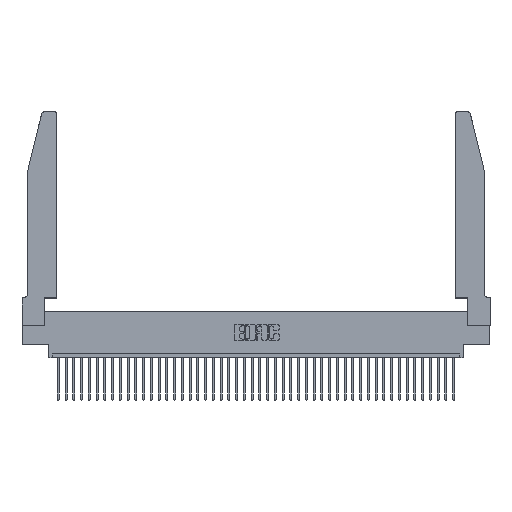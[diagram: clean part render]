
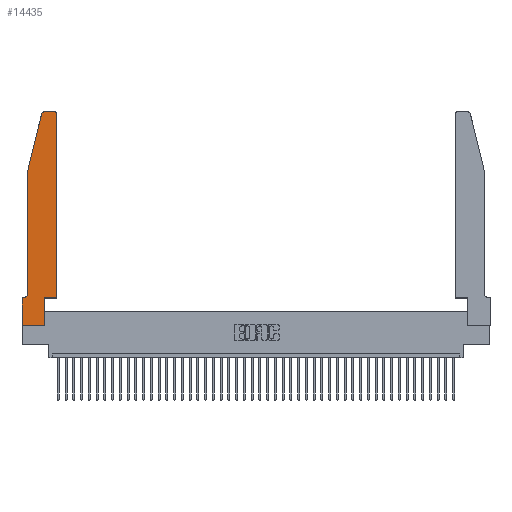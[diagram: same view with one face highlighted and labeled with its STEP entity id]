
A CAD part, top view. The second image highlights one B-rep face of the part: STEP entity #14435.
In plain terms, the highlighted planar face has unit normal (0, 0, 1).
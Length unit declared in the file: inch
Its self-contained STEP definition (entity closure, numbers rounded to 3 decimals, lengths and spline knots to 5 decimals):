
#172 = EDGE_CURVE ( 'NONE', #4846, #11020, #39690, .T. ) ;
#208 = VERTEX_POINT ( 'NONE', #11036 ) ;
#257 = VECTOR ( 'NONE', #23914, 39.37008 ) ;
#631 = VERTEX_POINT ( 'NONE', #15669 ) ;
#671 = EDGE_CURVE ( 'NONE', #29893, #631, #23609, .T. ) ;
#2301 = DIRECTION ( 'NONE',  ( -0.239, -0.971, 0. ) ) ;
#2379 = ORIENTED_EDGE ( 'NONE', *, *, #10121, .T. ) ;
#4210 = ORIENTED_EDGE ( 'NONE', *, *, #8724, .T. ) ;
#4527 = VERTEX_POINT ( 'NONE', #11928 ) ;
#4846 = VERTEX_POINT ( 'NONE', #10157 ) ;
#6494 = ORIENTED_EDGE ( 'NONE', *, *, #36489, .T. ) ;
#6908 = LINE ( 'NONE', #10457, #257 ) ;
#7983 = DIRECTION ( 'NONE',  ( -1., 0., 0. ) ) ;
#8712 = CARTESIAN_POINT ( 'NONE',  ( 0.0755, 2., 0.37 ) ) ;
#8724 = EDGE_CURVE ( 'NONE', #26366, #36573, #6908, .T. ) ;
#9397 = LINE ( 'NONE', #18089, #25946 ) ;
#9433 = EDGE_CURVE ( 'NONE', #10110, #4846, #27962, .T. ) ;
#10110 = VERTEX_POINT ( 'NONE', #39055 ) ;
#10121 = EDGE_CURVE ( 'NONE', #208, #10110, #38764, .T. ) ;
#10157 = CARTESIAN_POINT ( 'NONE',  ( 0., 0.35, 0.37 ) ) ;
#10457 = CARTESIAN_POINT ( 'NONE',  ( 0.4505, 0.35, 0.37 ) ) ;
#11008 = DIRECTION ( 'NONE',  ( 0., -1., 0. ) ) ;
#11020 = VERTEX_POINT ( 'NONE', #35320 ) ;
#11036 = CARTESIAN_POINT ( 'NONE',  ( 0.0755, 0.42, 0.37 ) ) ;
#11437 = CARTESIAN_POINT ( 'NONE',  ( 0.284, 2.72, 0.37 ) ) ;
#11928 = CARTESIAN_POINT ( 'NONE',  ( 0.284, 2.75, 0.37 ) ) ;
#12175 = ORIENTED_EDGE ( 'NONE', *, *, #34588, .T. ) ;
#12450 = VECTOR ( 'NONE', #26776, 39.37008 ) ;
#12914 = CARTESIAN_POINT ( 'NONE',  ( 0.4505, 0.35, 0.37 ) ) ;
#13186 = DIRECTION ( 'NONE',  ( 0., 0., 1. ) ) ;
#13796 = VECTOR ( 'NONE', #24364, 39.37008 ) ;
#14150 = AXIS2_PLACEMENT_3D ( 'NONE', #29646, #39798, #23182 ) ;
#14435 = ADVANCED_FACE ( 'NONE', ( #37259 ), #29930, .T. ) ;
#14663 = EDGE_CURVE ( 'NONE', #21038, #208, #38775, .T. ) ;
#14715 = CARTESIAN_POINT ( 'NONE',  ( 0.4205, 2.75, 0.37 ) ) ;
#14821 = AXIS2_PLACEMENT_3D ( 'NONE', #23727, #41196, #24897 ) ;
#15669 = CARTESIAN_POINT ( 'NONE',  ( 0.2865, 0.35, 0.37 ) ) ;
#16595 = VECTOR ( 'NONE', #2301, 39.37008 ) ;
#16760 = CARTESIAN_POINT ( 'NONE',  ( 0.0755, 0.35, 0.37 ) ) ;
#16885 = CARTESIAN_POINT ( 'NONE',  ( 0.4205, 2.72, 0.37 ) ) ;
#18067 = VECTOR ( 'NONE', #11008, 39.37008 ) ;
#18089 = CARTESIAN_POINT ( 'NONE',  ( 0.4505, 0.35, 0.37 ) ) ;
#19295 = LINE ( 'NONE', #35833, #41564 ) ;
#19531 = VECTOR ( 'NONE', #7983, 39.37008 ) ;
#19925 = EDGE_CURVE ( 'NONE', #11020, #29893, #19295, .T. ) ;
#20524 = ORIENTED_EDGE ( 'NONE', *, *, #42095, .T. ) ;
#20567 = CARTESIAN_POINT ( 'NONE',  ( 0., 0., 0.37 ) ) ;
#20759 = CARTESIAN_POINT ( 'NONE',  ( 0.0755, 2., 0.37 ) ) ;
#20807 = CARTESIAN_POINT ( 'NONE',  ( 0.4505, 2.72, 0.37 ) ) ;
#21038 = VERTEX_POINT ( 'NONE', #20759 ) ;
#21280 = CARTESIAN_POINT ( 'NONE',  ( 0.0755, 2., 0.37 ) ) ;
#21596 = VERTEX_POINT ( 'NONE', #39146 ) ;
#21988 = ORIENTED_EDGE ( 'NONE', *, *, #172, .T. ) ;
#22655 = LINE ( 'NONE', #41189, #19531 ) ;
#22909 = CARTESIAN_POINT ( 'NONE',  ( 0.2865, 0.35, 0.37 ) ) ;
#23182 = DIRECTION ( 'NONE',  ( 1., 0., 0. ) ) ;
#23219 = VERTEX_POINT ( 'NONE', #14715 ) ;
#23609 = LINE ( 'NONE', #22909, #35485 ) ;
#23727 = CARTESIAN_POINT ( 'NONE',  ( 0.0055, 0.42, 0.37 ) ) ;
#23914 = DIRECTION ( 'NONE',  ( 0., 1., 0. ) ) ;
#24216 = ORIENTED_EDGE ( 'NONE', *, *, #34265, .T. ) ;
#24364 = DIRECTION ( 'NONE',  ( 0., -1., 0. ) ) ;
#24897 = DIRECTION ( 'NONE',  ( -1., 0., 0. ) ) ;
#25946 = VECTOR ( 'NONE', #37589, 39.37008 ) ;
#26366 = VERTEX_POINT ( 'NONE', #12914 ) ;
#26776 = DIRECTION ( 'NONE',  ( -1., 0., 0. ) ) ;
#27962 = LINE ( 'NONE', #16760, #12450 ) ;
#28247 = EDGE_LOOP ( 'NONE', ( #41718, #20524, #24216, #42371, #2379, #41375, #21988, #41852, #39885, #12175, #4210, #6494 ) ) ;
#29340 = DIRECTION ( 'NONE',  ( 1., 0., 0. ) ) ;
#29646 = CARTESIAN_POINT ( 'NONE',  ( 0., 0.35, 0.37 ) ) ;
#29814 = DIRECTION ( 'NONE',  ( 0., 1., 0. ) ) ;
#29893 = VERTEX_POINT ( 'NONE', #42480 ) ;
#29930 = PLANE ( 'NONE',  #14150 ) ;
#30043 = LINE ( 'NONE', #8712, #16595 ) ;
#31474 = DIRECTION ( 'NONE',  ( 0., 0., 1. ) ) ;
#34265 = EDGE_CURVE ( 'NONE', #21596, #21038, #30043, .T. ) ;
#34524 = DIRECTION ( 'NONE',  ( 1., 0., 0. ) ) ;
#34588 = EDGE_CURVE ( 'NONE', #631, #26366, #9397, .T. ) ;
#34906 = CIRCLE ( 'NONE', #36586, 0.03 ) ;
#35320 = CARTESIAN_POINT ( 'NONE',  ( 0., 0., 0.37 ) ) ;
#35485 = VECTOR ( 'NONE', #29814, 39.37008 ) ;
#35833 = CARTESIAN_POINT ( 'NONE',  ( 0., 0., 0.37 ) ) ;
#36277 = DIRECTION ( 'NONE',  ( 1., 0., 0. ) ) ;
#36489 = EDGE_CURVE ( 'NONE', #36573, #23219, #41957, .T. ) ;
#36573 = VERTEX_POINT ( 'NONE', #20807 ) ;
#36586 = AXIS2_PLACEMENT_3D ( 'NONE', #11437, #31474, #34524 ) ;
#37259 = FACE_OUTER_BOUND ( 'NONE', #28247, .T. ) ;
#37295 = AXIS2_PLACEMENT_3D ( 'NONE', #16885, #13186, #36277 ) ;
#37589 = DIRECTION ( 'NONE',  ( 1., 0., 0. ) ) ;
#38070 = EDGE_CURVE ( 'NONE', #23219, #4527, #22655, .T. ) ;
#38764 = CIRCLE ( 'NONE', #14821, 0.07 ) ;
#38775 = LINE ( 'NONE', #21280, #18067 ) ;
#39055 = CARTESIAN_POINT ( 'NONE',  ( 0.0055, 0.35, 0.37 ) ) ;
#39146 = CARTESIAN_POINT ( 'NONE',  ( 0.25487, 2.72718, 0.37 ) ) ;
#39690 = LINE ( 'NONE', #20567, #13796 ) ;
#39798 = DIRECTION ( 'NONE',  ( 0., 0., 1. ) ) ;
#39885 = ORIENTED_EDGE ( 'NONE', *, *, #671, .T. ) ;
#41189 = CARTESIAN_POINT ( 'NONE',  ( 0.2605, 2.75, 0.37 ) ) ;
#41196 = DIRECTION ( 'NONE',  ( 0., 0., -1. ) ) ;
#41375 = ORIENTED_EDGE ( 'NONE', *, *, #9433, .T. ) ;
#41564 = VECTOR ( 'NONE', #29340, 39.37008 ) ;
#41718 = ORIENTED_EDGE ( 'NONE', *, *, #38070, .T. ) ;
#41852 = ORIENTED_EDGE ( 'NONE', *, *, #19925, .T. ) ;
#41957 = CIRCLE ( 'NONE', #37295, 0.03 ) ;
#42095 = EDGE_CURVE ( 'NONE', #4527, #21596, #34906, .T. ) ;
#42371 = ORIENTED_EDGE ( 'NONE', *, *, #14663, .T. ) ;
#42480 = CARTESIAN_POINT ( 'NONE',  ( 0.2865, 0., 0.37 ) ) ;
